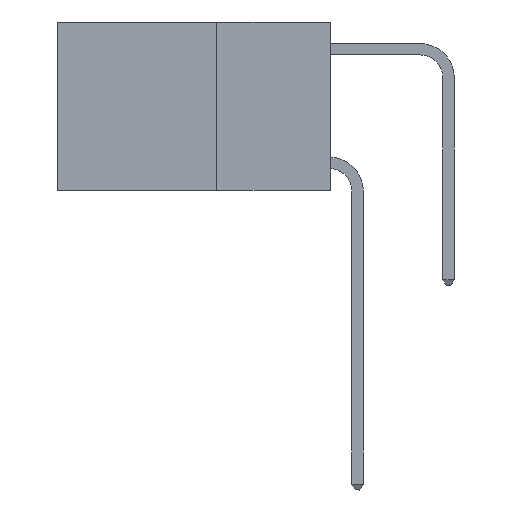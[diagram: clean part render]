
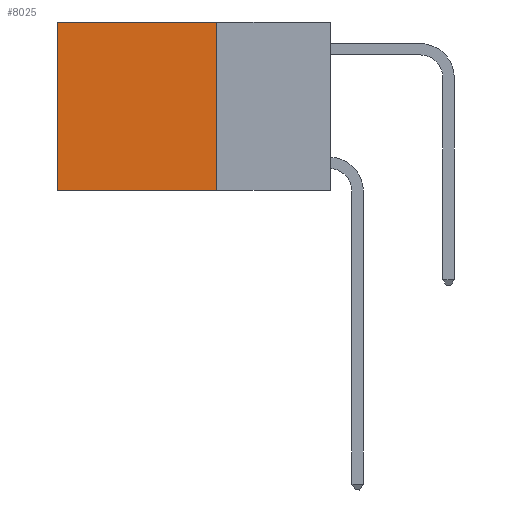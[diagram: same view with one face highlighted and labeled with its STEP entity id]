
A CAD part, left-side view. The second image highlights one B-rep face of the part: STEP entity #8025.
In plain terms, the highlighted planar face has unit normal (-1, 0, 0).
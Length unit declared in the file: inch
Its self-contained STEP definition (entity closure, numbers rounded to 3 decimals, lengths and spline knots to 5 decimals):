
#93 = EDGE_CURVE ( 'NONE', #808, #16767, #13672, .T. ) ;
#524 = CARTESIAN_POINT ( 'NONE',  ( 0.2625, 0.25, 0. ) ) ;
#808 = VERTEX_POINT ( 'NONE', #14408 ) ;
#876 = CARTESIAN_POINT ( 'NONE',  ( 0.2625, 0.25, 0. ) ) ;
#1933 = DIRECTION ( 'NONE',  ( 0., 0., -1. ) ) ;
#1940 = AXIS2_PLACEMENT_3D ( 'NONE', #524, #10007, #1933 ) ;
#2089 = CARTESIAN_POINT ( 'NONE',  ( 0.2625, 0.25, 0. ) ) ;
#2098 = LINE ( 'NONE', #4934, #8046 ) ;
#2282 = DIRECTION ( 'NONE',  ( 0., 0., -1. ) ) ;
#3465 = DIRECTION ( 'NONE',  ( 0., 1., 0. ) ) ;
#4589 = ORIENTED_EDGE ( 'NONE', *, *, #11767, .F. ) ;
#4625 = DIRECTION ( 'NONE',  ( 0., 1., 0. ) ) ;
#4703 = ORIENTED_EDGE ( 'NONE', *, *, #15738, .T. ) ;
#4934 = CARTESIAN_POINT ( 'NONE',  ( 0.2625, 0.25, -0.37 ) ) ;
#4991 = VECTOR ( 'NONE', #3465, 39.37008 ) ;
#6825 = EDGE_LOOP ( 'NONE', ( #16952, #4589, #7689, #4703 ) ) ;
#6997 = CARTESIAN_POINT ( 'NONE',  ( 0.2625, 0.6, -0.37 ) ) ;
#7663 = VECTOR ( 'NONE', #2282, 39.37008 ) ;
#7689 = ORIENTED_EDGE ( 'NONE', *, *, #17113, .F. ) ;
#7865 = DIRECTION ( 'NONE',  ( 0., 0., -1. ) ) ;
#8025 = ADVANCED_FACE ( 'NONE', ( #16328 ), #8681, .F. ) ;
#8046 = VECTOR ( 'NONE', #4625, 39.37008 ) ;
#8077 = LINE ( 'NONE', #876, #7663 ) ;
#8681 = PLANE ( 'NONE',  #1940 ) ;
#10007 = DIRECTION ( 'NONE',  ( 1., 0., 0. ) ) ;
#10485 = VERTEX_POINT ( 'NONE', #15311 ) ;
#11767 = EDGE_CURVE ( 'NONE', #15995, #16767, #2098, .T. ) ;
#12025 = CARTESIAN_POINT ( 'NONE',  ( 0.2625, 0.25, -0.37 ) ) ;
#12033 = CARTESIAN_POINT ( 'NONE',  ( 0.2625, 0.6, 0. ) ) ;
#13672 = LINE ( 'NONE', #12033, #15917 ) ;
#14408 = CARTESIAN_POINT ( 'NONE',  ( 0.2625, 0.6, 0. ) ) ;
#15311 = CARTESIAN_POINT ( 'NONE',  ( 0.2625, 0.25, 0. ) ) ;
#15548 = LINE ( 'NONE', #2089, #4991 ) ;
#15738 = EDGE_CURVE ( 'NONE', #10485, #808, #15548, .T. ) ;
#15917 = VECTOR ( 'NONE', #7865, 39.37008 ) ;
#15995 = VERTEX_POINT ( 'NONE', #12025 ) ;
#16328 = FACE_OUTER_BOUND ( 'NONE', #6825, .T. ) ;
#16767 = VERTEX_POINT ( 'NONE', #6997 ) ;
#16952 = ORIENTED_EDGE ( 'NONE', *, *, #93, .T. ) ;
#17113 = EDGE_CURVE ( 'NONE', #10485, #15995, #8077, .T. ) ;
